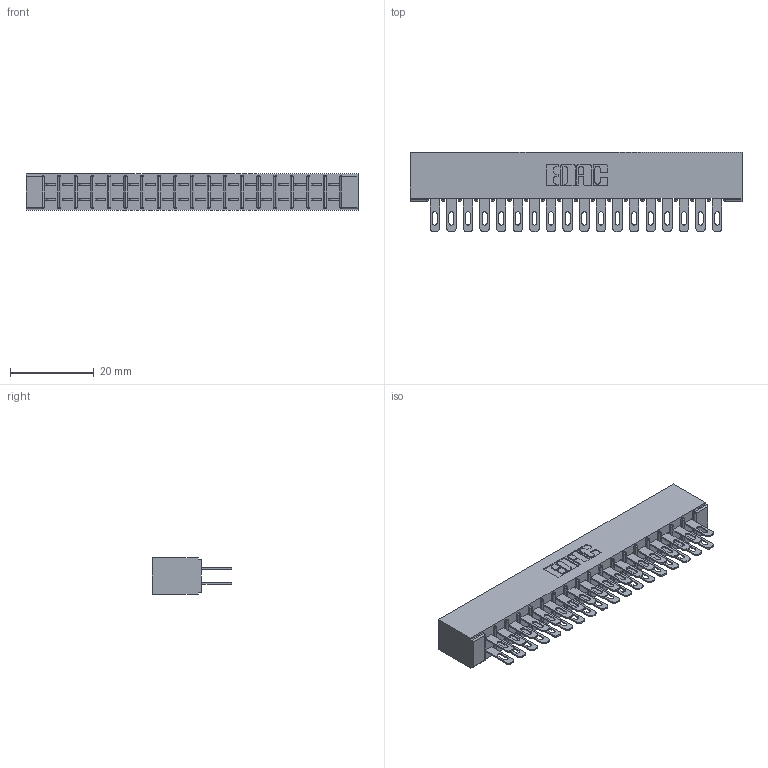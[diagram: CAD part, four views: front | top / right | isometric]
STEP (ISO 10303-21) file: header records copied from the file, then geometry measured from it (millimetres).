
FILE_DESCRIPTION (( 'STEP AP203' ), '1' );
FILE_NAME ('355-036-500-201.STEP', '2019-09-11T09:14:20', ( '' ), ( '' ), 'SwSTEP 2.0', 'SolidWorks 2016', '' );
FILE_SCHEMA (( 'CONFIG_CONTROL_DESIGN' ));
Length unit declared in the file: inch
Products named in the file (3): 305-290-001_500; 355-036-500-201; 305 Part_No Mounting
Assembly tree (37 placements, depth 2):
  355-036-500-201
    305 Part_No Mounting
    305-290-001_500  x36
Bounding box: 79.2 x 18.85 x 8.71 mm (x, y, z)
Volume: 5271 mm3; surface area: 10928.5 mm2
Topology: 37 solids, 37 shells, 1908 faces, 5458 edges, 3540 vertices
Faces by surface type: plane 1072, cylinder 764, sphere 72
Entity records: 22155 total; most frequent: CARTESIAN_POINT 3664, ORIENTED_EDGE 3632, DIRECTION 3564, EDGE_CURVE 1816, VECTOR 1444, LINE 1444, VERTEX_POINT 1160, AXIS2_PLACEMENT_3D 1060
